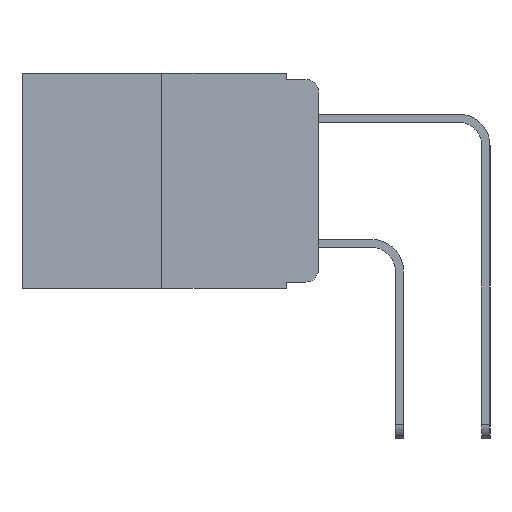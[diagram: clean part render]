
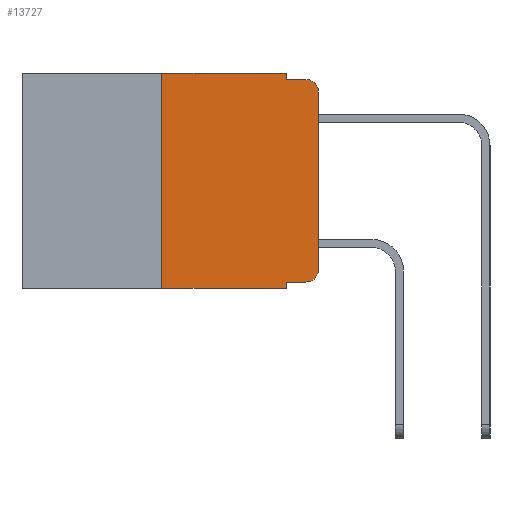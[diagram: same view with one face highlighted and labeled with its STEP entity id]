
A CAD part, left-side view. The second image highlights one B-rep face of the part: STEP entity #13727.
In plain terms, the highlighted planar face has unit normal (-1, 0, 0).
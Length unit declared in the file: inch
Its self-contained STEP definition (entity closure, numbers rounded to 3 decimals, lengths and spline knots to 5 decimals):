
#194 = VERTEX_POINT ( 'NONE', #4914 ) ;
#227 = EDGE_LOOP ( 'NONE', ( #5711, #9068, #4945, #10175, #15107, #5205, #13551, #14976, #1866, #12266 ) ) ;
#693 = DIRECTION ( 'NONE',  ( 0., -1., 0. ) ) ;
#853 = CARTESIAN_POINT ( 'NONE',  ( 0., 0.051, 0. ) ) ;
#906 = DIRECTION ( 'NONE',  ( 1., 0., 0. ) ) ;
#1117 = VERTEX_POINT ( 'NONE', #5933 ) ;
#1190 = DIRECTION ( 'NONE',  ( 0., 0., -1. ) ) ;
#1273 = VECTOR ( 'NONE', #14963, 39.37008 ) ;
#1374 = DIRECTION ( 'NONE',  ( -1., 0., 0. ) ) ;
#1487 = DIRECTION ( 'NONE',  ( 0., 0., -1. ) ) ;
#1723 = EDGE_CURVE ( 'NONE', #9771, #7034, #13810, .T. ) ;
#1757 = VERTEX_POINT ( 'NONE', #14353 ) ;
#1764 = DIRECTION ( 'NONE',  ( 0., -1., 0. ) ) ;
#1866 = ORIENTED_EDGE ( 'NONE', *, *, #15356, .T. ) ;
#2053 = VECTOR ( 'NONE', #14580, 39.37008 ) ;
#2290 = AXIS2_PLACEMENT_3D ( 'NONE', #15112, #906, #9325 ) ;
#2415 = LINE ( 'NONE', #5146, #2053 ) ;
#2830 = DIRECTION ( 'NONE',  ( 0., -1., 0. ) ) ;
#3152 = LINE ( 'NONE', #10615, #14968 ) ;
#3365 = CARTESIAN_POINT ( 'NONE',  ( 0., 0.02, -0.313 ) ) ;
#3620 = CARTESIAN_POINT ( 'NONE',  ( 0., 0.473, 0. ) ) ;
#3689 = AXIS2_PLACEMENT_3D ( 'NONE', #13183, #6104, #14338 ) ;
#4182 = EDGE_CURVE ( 'NONE', #9835, #194, #11198, .T. ) ;
#4240 = VECTOR ( 'NONE', #1487, 39.37008 ) ;
#4470 = LINE ( 'NONE', #3620, #1273 ) ;
#4689 = EDGE_CURVE ( 'NONE', #7623, #11912, #4470, .T. ) ;
#4860 = VECTOR ( 'NONE', #1764, 39.37008 ) ;
#4914 = CARTESIAN_POINT ( 'NONE',  ( 0., 0.02, -0.01 ) ) ;
#4945 = ORIENTED_EDGE ( 'NONE', *, *, #4182, .F. ) ;
#5146 = CARTESIAN_POINT ( 'NONE',  ( 0., 0.25, 0. ) ) ;
#5205 = ORIENTED_EDGE ( 'NONE', *, *, #13432, .F. ) ;
#5351 = LINE ( 'NONE', #8850, #5742 ) ;
#5459 = CARTESIAN_POINT ( 'NONE',  ( 0., 0.02, -0.333 ) ) ;
#5660 = EDGE_CURVE ( 'NONE', #14834, #1117, #12811, .T. ) ;
#5711 = ORIENTED_EDGE ( 'NONE', *, *, #11665, .T. ) ;
#5742 = VECTOR ( 'NONE', #2830, 39.37008 ) ;
#5813 = EDGE_CURVE ( 'NONE', #11912, #9835, #10606, .T. ) ;
#5933 = CARTESIAN_POINT ( 'NONE',  ( 0., 0., -0.313 ) ) ;
#6104 = DIRECTION ( 'NONE',  ( -1., 0., 0. ) ) ;
#6597 = CARTESIAN_POINT ( 'NONE',  ( 0., 0.051, -0.01 ) ) ;
#6601 = CARTESIAN_POINT ( 'NONE',  ( 0., 0., 0. ) ) ;
#6955 = PLANE ( 'NONE',  #2290 ) ;
#7034 = VERTEX_POINT ( 'NONE', #12503 ) ;
#7107 = DIRECTION ( 'NONE',  ( 0., 0., -1. ) ) ;
#7165 = CARTESIAN_POINT ( 'NONE',  ( 0., 0., -0.03 ) ) ;
#7592 = CARTESIAN_POINT ( 'NONE',  ( 0., 0.25, 0. ) ) ;
#7623 = VERTEX_POINT ( 'NONE', #7592 ) ;
#8040 = VERTEX_POINT ( 'NONE', #7165 ) ;
#8607 = CIRCLE ( 'NONE', #3689, 0.02 ) ;
#8850 = CARTESIAN_POINT ( 'NONE',  ( 0., 0.051, -0.333 ) ) ;
#8952 = CARTESIAN_POINT ( 'NONE',  ( 0., 0.473, -0.343 ) ) ;
#9068 = ORIENTED_EDGE ( 'NONE', *, *, #13230, .T. ) ;
#9325 = DIRECTION ( 'NONE',  ( 0., 0., -1. ) ) ;
#9771 = VERTEX_POINT ( 'NONE', #13574 ) ;
#9835 = VERTEX_POINT ( 'NONE', #12568 ) ;
#10175 = ORIENTED_EDGE ( 'NONE', *, *, #5813, .F. ) ;
#10606 = LINE ( 'NONE', #12597, #4240 ) ;
#10615 = CARTESIAN_POINT ( 'NONE',  ( 0., 0.051, 0. ) ) ;
#10629 = FACE_OUTER_BOUND ( 'NONE', #227, .T. ) ;
#10710 = VECTOR ( 'NONE', #693, 39.37008 ) ;
#11198 = LINE ( 'NONE', #6597, #4860 ) ;
#11665 = EDGE_CURVE ( 'NONE', #1117, #8040, #12094, .T. ) ;
#11912 = VERTEX_POINT ( 'NONE', #853 ) ;
#12094 = LINE ( 'NONE', #6601, #15156 ) ;
#12266 = ORIENTED_EDGE ( 'NONE', *, *, #5660, .T. ) ;
#12503 = CARTESIAN_POINT ( 'NONE',  ( 0., 0.051, -0.343 ) ) ;
#12568 = CARTESIAN_POINT ( 'NONE',  ( 0., 0.051, -0.01 ) ) ;
#12597 = CARTESIAN_POINT ( 'NONE',  ( 0., 0.051, 0. ) ) ;
#12811 = CIRCLE ( 'NONE', #13252, 0.02 ) ;
#13183 = CARTESIAN_POINT ( 'NONE',  ( 0., 0.02, -0.03 ) ) ;
#13230 = EDGE_CURVE ( 'NONE', #8040, #194, #8607, .T. ) ;
#13252 = AXIS2_PLACEMENT_3D ( 'NONE', #3365, #1374, #1190 ) ;
#13432 = EDGE_CURVE ( 'NONE', #9771, #7623, #2415, .T. ) ;
#13551 = ORIENTED_EDGE ( 'NONE', *, *, #1723, .T. ) ;
#13574 = CARTESIAN_POINT ( 'NONE',  ( 0., 0.25, -0.343 ) ) ;
#13727 = ADVANCED_FACE ( 'NONE', ( #10629 ), #6955, .F. ) ;
#13810 = LINE ( 'NONE', #8952, #10710 ) ;
#13828 = EDGE_CURVE ( 'NONE', #1757, #7034, #3152, .T. ) ;
#14338 = DIRECTION ( 'NONE',  ( 0., 0., -1. ) ) ;
#14353 = CARTESIAN_POINT ( 'NONE',  ( 0., 0.051, -0.333 ) ) ;
#14580 = DIRECTION ( 'NONE',  ( 0., 0., 1. ) ) ;
#14789 = DIRECTION ( 'NONE',  ( 0., 0., 1. ) ) ;
#14834 = VERTEX_POINT ( 'NONE', #5459 ) ;
#14963 = DIRECTION ( 'NONE',  ( 0., -1., 0. ) ) ;
#14968 = VECTOR ( 'NONE', #7107, 39.37008 ) ;
#14976 = ORIENTED_EDGE ( 'NONE', *, *, #13828, .F. ) ;
#15107 = ORIENTED_EDGE ( 'NONE', *, *, #4689, .F. ) ;
#15112 = CARTESIAN_POINT ( 'NONE',  ( 0., 0.473, 0. ) ) ;
#15156 = VECTOR ( 'NONE', #14789, 39.37008 ) ;
#15356 = EDGE_CURVE ( 'NONE', #1757, #14834, #5351, .T. ) ;
